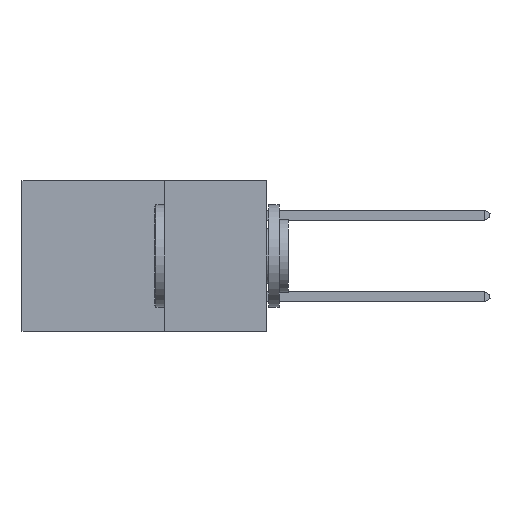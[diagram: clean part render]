
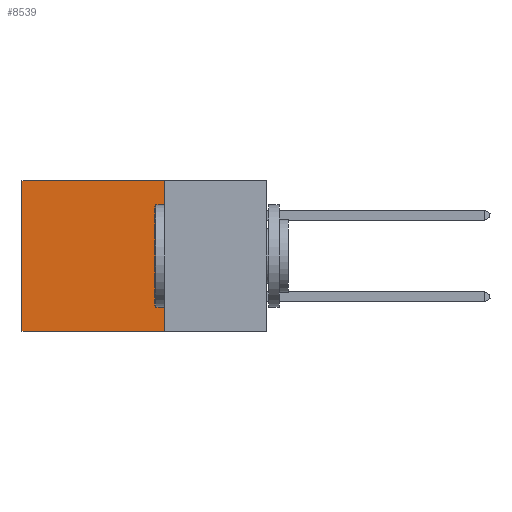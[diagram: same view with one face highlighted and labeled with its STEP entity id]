
A CAD part, left-side view. The second image highlights one B-rep face of the part: STEP entity #8539.
In plain terms, the highlighted planar face has unit normal (-1, 0, 0).
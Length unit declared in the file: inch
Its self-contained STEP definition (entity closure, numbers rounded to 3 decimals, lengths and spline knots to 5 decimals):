
#163 = EDGE_CURVE ( 'NONE', #9211, #4636, #12094, .T. ) ;
#171 = FACE_OUTER_BOUND ( 'NONE', #10104, .T. ) ;
#310 = ORIENTED_EDGE ( 'NONE', *, *, #9548, .T. ) ;
#682 = CARTESIAN_POINT ( 'NONE',  ( 0.2875, 0.6, -0.37 ) ) ;
#986 = CARTESIAN_POINT ( 'NONE',  ( 0.2875, 0.6, 0. ) ) ;
#1329 = CARTESIAN_POINT ( 'NONE',  ( 0.2875, 0.25, 0. ) ) ;
#1666 = DIRECTION ( 'NONE',  ( 1., 0., 0. ) ) ;
#1671 = VERTEX_POINT ( 'NONE', #3903 ) ;
#2094 = EDGE_CURVE ( 'NONE', #7452, #1671, #6745, .T. ) ;
#3314 = DIRECTION ( 'NONE',  ( 0., 0., -1. ) ) ;
#3594 = CARTESIAN_POINT ( 'NONE',  ( 0.2875, 0.25, 0. ) ) ;
#3903 = CARTESIAN_POINT ( 'NONE',  ( 0.2875, 0.25, -0.37 ) ) ;
#3991 = CARTESIAN_POINT ( 'NONE',  ( 0.2875, 0.25, 0. ) ) ;
#4385 = CARTESIAN_POINT ( 'NONE',  ( 0.2875, 0.25, -0.37 ) ) ;
#4636 = VERTEX_POINT ( 'NONE', #682 ) ;
#4640 = VECTOR ( 'NONE', #4966, 39.37008 ) ;
#4966 = DIRECTION ( 'NONE',  ( 0., 1., 0. ) ) ;
#4976 = VECTOR ( 'NONE', #3314, 39.37008 ) ;
#5214 = EDGE_CURVE ( 'NONE', #1671, #4636, #9044, .T. ) ;
#5356 = ORIENTED_EDGE ( 'NONE', *, *, #163, .T. ) ;
#6166 = VECTOR ( 'NONE', #7582, 39.37008 ) ;
#6674 = VECTOR ( 'NONE', #8105, 39.37008 ) ;
#6745 = LINE ( 'NONE', #7804, #6166 ) ;
#7398 = PLANE ( 'NONE',  #11232 ) ;
#7452 = VERTEX_POINT ( 'NONE', #1329 ) ;
#7582 = DIRECTION ( 'NONE',  ( 0., 0., -1. ) ) ;
#7798 = ORIENTED_EDGE ( 'NONE', *, *, #5214, .F. ) ;
#7804 = CARTESIAN_POINT ( 'NONE',  ( 0.2875, 0.25, 0. ) ) ;
#8105 = DIRECTION ( 'NONE',  ( 0., 1., 0. ) ) ;
#8269 = DIRECTION ( 'NONE',  ( 0., 0., -1. ) ) ;
#8539 = ADVANCED_FACE ( 'NONE', ( #171 ), #7398, .F. ) ;
#9044 = LINE ( 'NONE', #4385, #6674 ) ;
#9211 = VERTEX_POINT ( 'NONE', #11749 ) ;
#9548 = EDGE_CURVE ( 'NONE', #7452, #9211, #11807, .T. ) ;
#10104 = EDGE_LOOP ( 'NONE', ( #5356, #7798, #10158, #310 ) ) ;
#10158 = ORIENTED_EDGE ( 'NONE', *, *, #2094, .F. ) ;
#11232 = AXIS2_PLACEMENT_3D ( 'NONE', #3594, #1666, #8269 ) ;
#11749 = CARTESIAN_POINT ( 'NONE',  ( 0.2875, 0.6, 0. ) ) ;
#11807 = LINE ( 'NONE', #3991, #4640 ) ;
#12094 = LINE ( 'NONE', #986, #4976 ) ;
